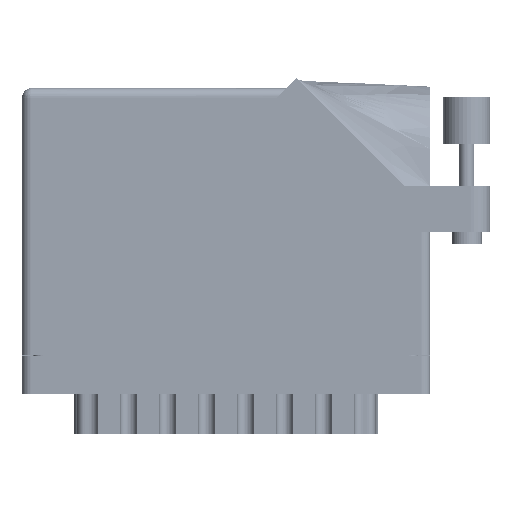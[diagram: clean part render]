
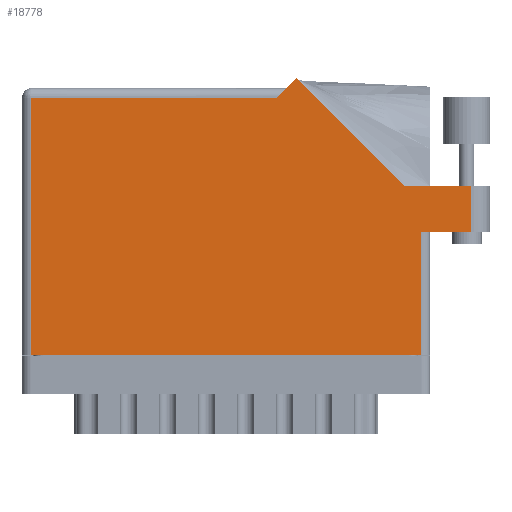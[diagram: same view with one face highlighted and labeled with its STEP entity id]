
A CAD part, front view. The second image highlights one B-rep face of the part: STEP entity #18778.
In plain terms, the highlighted face is planar.
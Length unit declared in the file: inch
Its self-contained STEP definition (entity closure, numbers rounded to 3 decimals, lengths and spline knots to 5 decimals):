
#1469 = VECTOR ( 'NONE', #30915, 39.37008 ) ;
#1503 = LINE ( 'NONE', #71635, #31427 ) ;
#2204 = ORIENTED_EDGE ( 'NONE', *, *, #2479, .T. ) ;
#2479 = EDGE_CURVE ( 'NONE', #14078, #63622, #1503, .T. ) ;
#3322 = VERTEX_POINT ( 'NONE', #11801 ) ;
#3493 = AXIS2_PLACEMENT_3D ( 'NONE', #19676, #20438, #61881 ) ;
#5080 = EDGE_CURVE ( 'NONE', #24712, #38966, #14399, .T. ) ;
#5294 = EDGE_CURVE ( 'NONE', #59545, #3322, #66773, .T. ) ;
#7514 = DIRECTION ( 'NONE',  ( -1., 0., 0. ) ) ;
#10834 = ORIENTED_EDGE ( 'NONE', *, *, #5080, .T. ) ;
#11801 = CARTESIAN_POINT ( 'NONE',  ( 0.062, 1.713, 0. ) ) ;
#14078 = VERTEX_POINT ( 'NONE', #18545 ) ;
#14399 = LINE ( 'NONE', #61640, #36831 ) ;
#16695 = VECTOR ( 'NONE', #32837, 39.37008 ) ;
#18545 = CARTESIAN_POINT ( 'NONE',  ( 0.062, 0., 0. ) ) ;
#18778 = ADVANCED_FACE ( 'NONE', ( #43305 ), #43681, .F. ) ;
#19676 = CARTESIAN_POINT ( 'NONE',  ( 0., 1.775, 0. ) ) ;
#20438 = DIRECTION ( 'NONE',  ( 0., 0., -1. ) ) ;
#20550 = EDGE_CURVE ( 'NONE', #63622, #62031, #54050, .T. ) ;
#21468 = CARTESIAN_POINT ( 'NONE',  ( 2.55242, 1.122, 0. ) ) ;
#23704 = CARTESIAN_POINT ( 'NONE',  ( 2.656, 0., 0. ) ) ;
#23930 = VECTOR ( 'NONE', #7514, 39.37008 ) ;
#24176 = CARTESIAN_POINT ( 'NONE',  ( 2.656, 0.815, 0. ) ) ;
#24712 = VERTEX_POINT ( 'NONE', #41180 ) ;
#25091 = CARTESIAN_POINT ( 'NONE',  ( 0.062, 0., 0. ) ) ;
#26141 = DIRECTION ( 'NONE',  ( -0.707, 0.707, 0. ) ) ;
#26358 = DIRECTION ( 'NONE',  ( 1., 0., 0. ) ) ;
#26958 = VERTEX_POINT ( 'NONE', #57940 ) ;
#27374 = CARTESIAN_POINT ( 'NONE',  ( 1.758, 1.775, 0. ) ) ;
#29763 = LINE ( 'NONE', #25091, #1469 ) ;
#30915 = DIRECTION ( 'NONE',  ( 0., -1., 0. ) ) ;
#31186 = CARTESIAN_POINT ( 'NONE',  ( 2.656, 0.815, 0. ) ) ;
#31427 = VECTOR ( 'NONE', #72403, 39.37008 ) ;
#31775 = CARTESIAN_POINT ( 'NONE',  ( 2.55242, 1.122, 0. ) ) ;
#32205 = VERTEX_POINT ( 'NONE', #31775 ) ;
#32837 = DIRECTION ( 'NONE',  ( -0.707, -0.707, 0. ) ) ;
#33120 = LINE ( 'NONE', #21468, #44447 ) ;
#33169 = ORIENTED_EDGE ( 'NONE', *, *, #42905, .T. ) ;
#35990 = DIRECTION ( 'NONE',  ( 0., 1., 0. ) ) ;
#36350 = ORIENTED_EDGE ( 'NONE', *, *, #43662, .T. ) ;
#36831 = VECTOR ( 'NONE', #35990, 39.37008 ) ;
#37582 = VECTOR ( 'NONE', #43185, 39.37008 ) ;
#37603 = DIRECTION ( 'NONE',  ( -1., 0., 0. ) ) ;
#38395 = CARTESIAN_POINT ( 'NONE',  ( 2.718, 0.815, 0. ) ) ;
#38966 = VERTEX_POINT ( 'NONE', #60855 ) ;
#41180 = CARTESIAN_POINT ( 'NONE',  ( 2.993, 0.815, 0. ) ) ;
#42645 = LINE ( 'NONE', #47714, #45768 ) ;
#42905 = EDGE_CURVE ( 'NONE', #62031, #24712, #73250, .T. ) ;
#43185 = DIRECTION ( 'NONE',  ( 0., 1., 0. ) ) ;
#43305 = FACE_OUTER_BOUND ( 'NONE', #44797, .T. ) ;
#43662 = EDGE_CURVE ( 'NONE', #32205, #26958, #33120, .T. ) ;
#43681 = PLANE ( 'NONE',  #3493 ) ;
#43803 = EDGE_CURVE ( 'NONE', #38966, #32205, #42645, .T. ) ;
#44447 = VECTOR ( 'NONE', #26141, 39.37008 ) ;
#44797 = EDGE_LOOP ( 'NONE', ( #33169, #10834, #52210, #36350, #69183, #47436, #66032, #2204, #53562 ) ) ;
#45236 = CARTESIAN_POINT ( 'NONE',  ( 1.696, 1.713, 0. ) ) ;
#45768 = VECTOR ( 'NONE', #37603, 39.37008 ) ;
#47436 = ORIENTED_EDGE ( 'NONE', *, *, #5294, .T. ) ;
#47714 = CARTESIAN_POINT ( 'NONE',  ( 3.118, 1.122, 0. ) ) ;
#49493 = LINE ( 'NONE', #27374, #16695 ) ;
#52210 = ORIENTED_EDGE ( 'NONE', *, *, #43803, .T. ) ;
#53562 = ORIENTED_EDGE ( 'NONE', *, *, #20550, .T. ) ;
#54050 = LINE ( 'NONE', #31186, #37582 ) ;
#56461 = EDGE_CURVE ( 'NONE', #26958, #59545, #49493, .T. ) ;
#57940 = CARTESIAN_POINT ( 'NONE',  ( 1.82871, 1.84571, 0. ) ) ;
#59545 = VERTEX_POINT ( 'NONE', #45236 ) ;
#60855 = CARTESIAN_POINT ( 'NONE',  ( 2.993, 1.122, 0. ) ) ;
#61640 = CARTESIAN_POINT ( 'NONE',  ( 2.993, 1.122, 0. ) ) ;
#61881 = DIRECTION ( 'NONE',  ( -1., 0., 0. ) ) ;
#62031 = VERTEX_POINT ( 'NONE', #24176 ) ;
#63622 = VERTEX_POINT ( 'NONE', #23704 ) ;
#64353 = VECTOR ( 'NONE', #26358, 39.37008 ) ;
#65266 = CARTESIAN_POINT ( 'NONE',  ( 0., 1.713, 0. ) ) ;
#66032 = ORIENTED_EDGE ( 'NONE', *, *, #75322, .T. ) ;
#66773 = LINE ( 'NONE', #65266, #23930 ) ;
#69183 = ORIENTED_EDGE ( 'NONE', *, *, #56461, .T. ) ;
#71635 = CARTESIAN_POINT ( 'NONE',  ( 0., 0., 0. ) ) ;
#72403 = DIRECTION ( 'NONE',  ( 1., 0., 0. ) ) ;
#73250 = LINE ( 'NONE', #38395, #64353 ) ;
#75322 = EDGE_CURVE ( 'NONE', #3322, #14078, #29763, .T. ) ;
